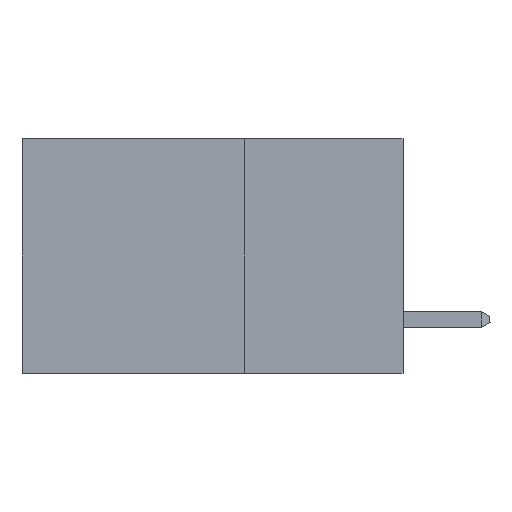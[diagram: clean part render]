
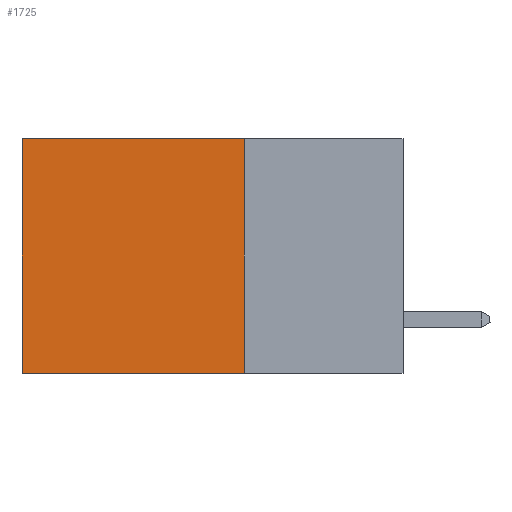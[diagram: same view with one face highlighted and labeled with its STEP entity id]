
A CAD part, left-side view. The second image highlights one B-rep face of the part: STEP entity #1725.
In plain terms, the highlighted planar face has unit normal (-1, 0, 0).
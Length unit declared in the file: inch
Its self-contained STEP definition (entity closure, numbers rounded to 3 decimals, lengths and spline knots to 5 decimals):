
#1122 = VECTOR ( 'NONE', #10228, 39.37008 ) ;
#1725 = ADVANCED_FACE ( 'NONE', ( #42373 ), #33786, .F. ) ;
#1970 = EDGE_CURVE ( 'NONE', #41715, #17918, #15598, .T. ) ;
#3783 = EDGE_CURVE ( 'NONE', #41715, #23225, #20356, .T. ) ;
#5602 = LINE ( 'NONE', #26943, #15975 ) ;
#6748 = CARTESIAN_POINT ( 'NONE',  ( 0.2875, 0.6, 0. ) ) ;
#9103 = EDGE_CURVE ( 'NONE', #17918, #13326, #5602, .T. ) ;
#9982 = EDGE_CURVE ( 'NONE', #23225, #13326, #11493, .T. ) ;
#10228 = DIRECTION ( 'NONE',  ( 0., 0., -1. ) ) ;
#11493 = LINE ( 'NONE', #6748, #1122 ) ;
#12385 = DIRECTION ( 'NONE',  ( 0., 0., -1. ) ) ;
#13326 = VERTEX_POINT ( 'NONE', #43850 ) ;
#14734 = ORIENTED_EDGE ( 'NONE', *, *, #1970, .F. ) ;
#15598 = LINE ( 'NONE', #41644, #35237 ) ;
#15975 = VECTOR ( 'NONE', #20084, 39.37008 ) ;
#17918 = VERTEX_POINT ( 'NONE', #44382 ) ;
#18278 = CARTESIAN_POINT ( 'NONE',  ( 0.2875, 0.25, 0. ) ) ;
#19262 = CARTESIAN_POINT ( 'NONE',  ( 0.2875, 0.25, 0. ) ) ;
#20084 = DIRECTION ( 'NONE',  ( 0., 1., 0. ) ) ;
#20356 = LINE ( 'NONE', #18278, #40010 ) ;
#21632 = AXIS2_PLACEMENT_3D ( 'NONE', #19262, #37136, #12385 ) ;
#23225 = VERTEX_POINT ( 'NONE', #40084 ) ;
#23741 = DIRECTION ( 'NONE',  ( 0., 0., -1. ) ) ;
#25485 = CARTESIAN_POINT ( 'NONE',  ( 0.2875, 0.25, 0. ) ) ;
#26943 = CARTESIAN_POINT ( 'NONE',  ( 0.2875, 0.25, -0.37 ) ) ;
#27670 = ORIENTED_EDGE ( 'NONE', *, *, #3783, .T. ) ;
#33596 = DIRECTION ( 'NONE',  ( 0., 1., 0. ) ) ;
#33786 = PLANE ( 'NONE',  #21632 ) ;
#34679 = ORIENTED_EDGE ( 'NONE', *, *, #9103, .F. ) ;
#35237 = VECTOR ( 'NONE', #23741, 39.37008 ) ;
#37136 = DIRECTION ( 'NONE',  ( 1., 0., 0. ) ) ;
#40010 = VECTOR ( 'NONE', #33596, 39.37008 ) ;
#40084 = CARTESIAN_POINT ( 'NONE',  ( 0.2875, 0.6, 0. ) ) ;
#41103 = ORIENTED_EDGE ( 'NONE', *, *, #9982, .T. ) ;
#41644 = CARTESIAN_POINT ( 'NONE',  ( 0.2875, 0.25, 0. ) ) ;
#41715 = VERTEX_POINT ( 'NONE', #25485 ) ;
#42373 = FACE_OUTER_BOUND ( 'NONE', #45193, .T. ) ;
#43850 = CARTESIAN_POINT ( 'NONE',  ( 0.2875, 0.6, -0.37 ) ) ;
#44382 = CARTESIAN_POINT ( 'NONE',  ( 0.2875, 0.25, -0.37 ) ) ;
#45193 = EDGE_LOOP ( 'NONE', ( #41103, #34679, #14734, #27670 ) ) ;
